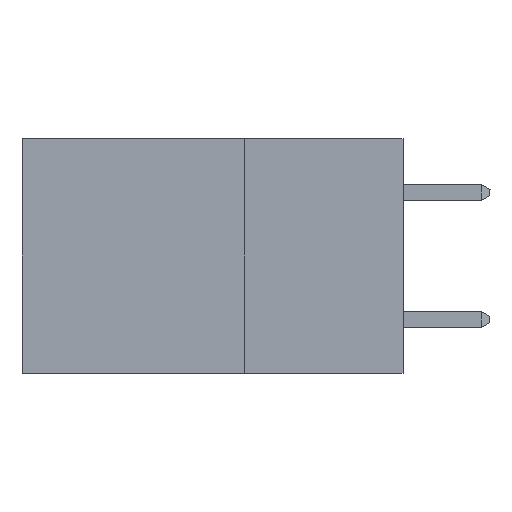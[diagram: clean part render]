
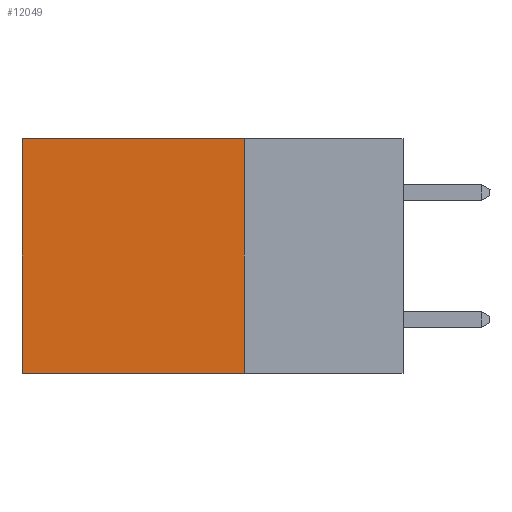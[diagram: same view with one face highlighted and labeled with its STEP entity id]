
A CAD part, left-side view. The second image highlights one B-rep face of the part: STEP entity #12049.
In plain terms, the highlighted planar face has unit normal (-1, 0, 0).
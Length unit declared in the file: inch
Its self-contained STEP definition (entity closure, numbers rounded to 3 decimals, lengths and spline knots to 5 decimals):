
#10 = CARTESIAN_POINT ( 'NONE',  ( 0.2875, 0.25, 0. ) ) ;
#415 = CARTESIAN_POINT ( 'NONE',  ( 0.2875, 0.6, 0. ) ) ;
#999 = CARTESIAN_POINT ( 'NONE',  ( 0.2875, 0.25, 0. ) ) ;
#1409 = VERTEX_POINT ( 'NONE', #10 ) ;
#1465 = PLANE ( 'NONE',  #24403 ) ;
#1606 = VECTOR ( 'NONE', #26304, 39.37008 ) ;
#2221 = VERTEX_POINT ( 'NONE', #28057 ) ;
#3152 = DIRECTION ( 'NONE',  ( 0., 1., 0. ) ) ;
#3639 = ORIENTED_EDGE ( 'NONE', *, *, #16741, .F. ) ;
#4400 = VERTEX_POINT ( 'NONE', #5017 ) ;
#5017 = CARTESIAN_POINT ( 'NONE',  ( 0.2875, 0.6, -0.37 ) ) ;
#6580 = EDGE_LOOP ( 'NONE', ( #8679, #3639, #21724, #22177 ) ) ;
#6686 = VERTEX_POINT ( 'NONE', #415 ) ;
#8679 = ORIENTED_EDGE ( 'NONE', *, *, #28919, .T. ) ;
#9219 = VECTOR ( 'NONE', #12219, 39.37008 ) ;
#9753 = FACE_OUTER_BOUND ( 'NONE', #6580, .T. ) ;
#10464 = DIRECTION ( 'NONE',  ( 1., 0., 0. ) ) ;
#10858 = VECTOR ( 'NONE', #28655, 39.37008 ) ;
#12040 = EDGE_CURVE ( 'NONE', #1409, #2221, #27754, .T. ) ;
#12049 = ADVANCED_FACE ( 'NONE', ( #9753 ), #1465, .F. ) ;
#12219 = DIRECTION ( 'NONE',  ( 0., 0., -1. ) ) ;
#12959 = DIRECTION ( 'NONE',  ( 0., 0., -1. ) ) ;
#15902 = LINE ( 'NONE', #999, #1606 ) ;
#16741 = EDGE_CURVE ( 'NONE', #2221, #4400, #19289, .T. ) ;
#18795 = CARTESIAN_POINT ( 'NONE',  ( 0.2875, 0.25, -0.37 ) ) ;
#18909 = LINE ( 'NONE', #23599, #9219 ) ;
#19289 = LINE ( 'NONE', #18795, #21091 ) ;
#21091 = VECTOR ( 'NONE', #3152, 39.37008 ) ;
#21724 = ORIENTED_EDGE ( 'NONE', *, *, #12040, .F. ) ;
#22177 = ORIENTED_EDGE ( 'NONE', *, *, #25093, .T. ) ;
#23599 = CARTESIAN_POINT ( 'NONE',  ( 0.2875, 0.6, 0. ) ) ;
#24403 = AXIS2_PLACEMENT_3D ( 'NONE', #26477, #10464, #12959 ) ;
#25093 = EDGE_CURVE ( 'NONE', #1409, #6686, #15902, .T. ) ;
#26304 = DIRECTION ( 'NONE',  ( 0., 1., 0. ) ) ;
#26477 = CARTESIAN_POINT ( 'NONE',  ( 0.2875, 0.25, 0. ) ) ;
#27754 = LINE ( 'NONE', #28334, #10858 ) ;
#28057 = CARTESIAN_POINT ( 'NONE',  ( 0.2875, 0.25, -0.37 ) ) ;
#28334 = CARTESIAN_POINT ( 'NONE',  ( 0.2875, 0.25, 0. ) ) ;
#28655 = DIRECTION ( 'NONE',  ( 0., 0., -1. ) ) ;
#28919 = EDGE_CURVE ( 'NONE', #6686, #4400, #18909, .T. ) ;
